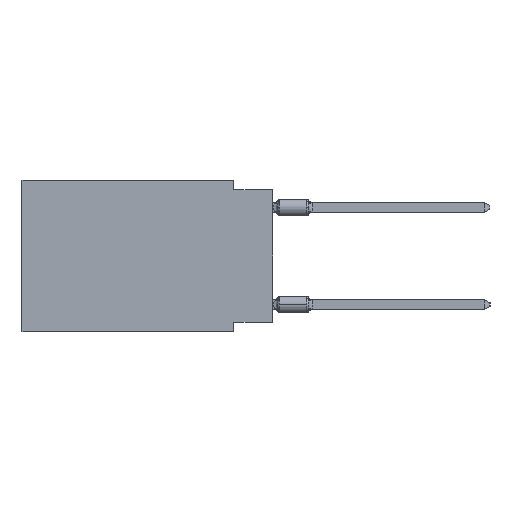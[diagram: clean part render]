
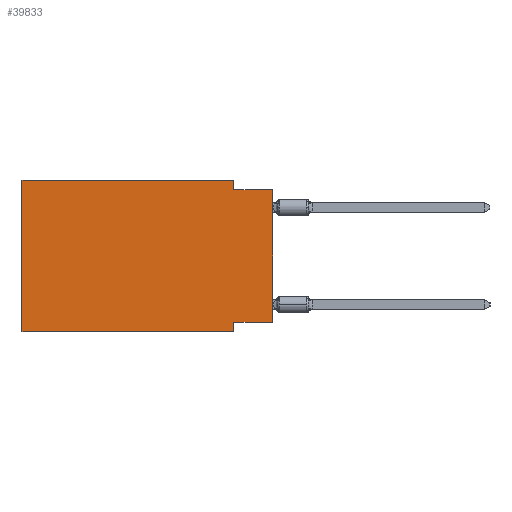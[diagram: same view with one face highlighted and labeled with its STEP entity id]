
A CAD part, left-side view. The second image highlights one B-rep face of the part: STEP entity #39833.
In plain terms, the highlighted planar face has unit normal (-1, 0, 0).
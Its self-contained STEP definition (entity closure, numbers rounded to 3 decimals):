
#191 = DIRECTION ( 'NONE',  ( 0., 0., 1. ) ) ;
#580 = ORIENTED_EDGE ( 'NONE', *, *, #36542, .F. ) ;
#1062 = ORIENTED_EDGE ( 'NONE', *, *, #32069, .F. ) ;
#1510 = FACE_OUTER_BOUND ( 'NONE', #15687, .T. ) ;
#2168 = CARTESIAN_POINT ( 'NONE',  ( 0., 16.383, 0. ) ) ;
#2452 = DIRECTION ( 'NONE',  ( 0., 0., 1. ) ) ;
#4817 = VECTOR ( 'NONE', #40927, 1000. ) ;
#5210 = AXIS2_PLACEMENT_3D ( 'NONE', #20588, #33257, #12476 ) ;
#7306 = DIRECTION ( 'NONE',  ( 0., -1., 0. ) ) ;
#7735 = CARTESIAN_POINT ( 'NONE',  ( 0., 2.54, -9.271 ) ) ;
#8302 = LINE ( 'NONE', #33609, #25710 ) ;
#9130 = VERTEX_POINT ( 'NONE', #20212 ) ;
#11033 = CARTESIAN_POINT ( 'NONE',  ( 0., 16.383, 0. ) ) ;
#11598 = EDGE_CURVE ( 'NONE', #34764, #33278, #39577, .T. ) ;
#11799 = CARTESIAN_POINT ( 'NONE',  ( 0., 0., 0. ) ) ;
#12476 = DIRECTION ( 'NONE',  ( 0., 0., -1. ) ) ;
#12644 = LINE ( 'NONE', #25909, #13486 ) ;
#13308 = ORIENTED_EDGE ( 'NONE', *, *, #27473, .T. ) ;
#13486 = VECTOR ( 'NONE', #191, 1000. ) ;
#14678 = CARTESIAN_POINT ( 'NONE',  ( 0., 2.54, 0. ) ) ;
#14810 = CARTESIAN_POINT ( 'NONE',  ( 0., 16.383, -9.906 ) ) ;
#15114 = LINE ( 'NONE', #11799, #21422 ) ;
#15620 = CARTESIAN_POINT ( 'NONE',  ( 0., 0., -9.271 ) ) ;
#15687 = EDGE_LOOP ( 'NONE', ( #13308, #1062, #30824, #21571, #31313, #17595, #580, #33397 ) ) ;
#16104 = EDGE_CURVE ( 'NONE', #22402, #34764, #26996, .T. ) ;
#16504 = CARTESIAN_POINT ( 'NONE',  ( 0., 0., -9.271 ) ) ;
#16979 = CARTESIAN_POINT ( 'NONE',  ( 0., 2.54, 0. ) ) ;
#17037 = VECTOR ( 'NONE', #30903, 1000. ) ;
#17595 = ORIENTED_EDGE ( 'NONE', *, *, #33598, .T. ) ;
#17702 = CARTESIAN_POINT ( 'NONE',  ( 0., 0., -0.635 ) ) ;
#18030 = VECTOR ( 'NONE', #21095, 1000. ) ;
#20212 = CARTESIAN_POINT ( 'NONE',  ( 0., 2.54, -9.906 ) ) ;
#20588 = CARTESIAN_POINT ( 'NONE',  ( 0., 16.383, 0. ) ) ;
#21095 = DIRECTION ( 'NONE',  ( 0., 0., -1. ) ) ;
#21422 = VECTOR ( 'NONE', #2452, 1000. ) ;
#21571 = ORIENTED_EDGE ( 'NONE', *, *, #16104, .F. ) ;
#21600 = VECTOR ( 'NONE', #7306, 1000. ) ;
#22402 = VERTEX_POINT ( 'NONE', #2168 ) ;
#25710 = VECTOR ( 'NONE', #33818, 1000. ) ;
#25831 = EDGE_CURVE ( 'NONE', #26641, #35912, #28277, .T. ) ;
#25909 = CARTESIAN_POINT ( 'NONE',  ( 0., 16.383, 0. ) ) ;
#26641 = VERTEX_POINT ( 'NONE', #16504 ) ;
#26996 = LINE ( 'NONE', #11033, #21600 ) ;
#27473 = EDGE_CURVE ( 'NONE', #26641, #30458, #15114, .T. ) ;
#27774 = VECTOR ( 'NONE', #29831, 1000. ) ;
#28253 = EDGE_CURVE ( 'NONE', #29119, #22402, #12644, .T. ) ;
#28277 = LINE ( 'NONE', #15620, #4817 ) ;
#28385 = LINE ( 'NONE', #14810, #27774 ) ;
#29119 = VERTEX_POINT ( 'NONE', #29334 ) ;
#29334 = CARTESIAN_POINT ( 'NONE',  ( 0., 16.383, -9.906 ) ) ;
#29831 = DIRECTION ( 'NONE',  ( 0., -1., 0. ) ) ;
#30458 = VERTEX_POINT ( 'NONE', #17702 ) ;
#30824 = ORIENTED_EDGE ( 'NONE', *, *, #11598, .F. ) ;
#30903 = DIRECTION ( 'NONE',  ( 0., 0., -1. ) ) ;
#31313 = ORIENTED_EDGE ( 'NONE', *, *, #28253, .F. ) ;
#32069 = EDGE_CURVE ( 'NONE', #33278, #30458, #8302, .T. ) ;
#33257 = DIRECTION ( 'NONE',  ( 1., 0., 0. ) ) ;
#33278 = VERTEX_POINT ( 'NONE', #36317 ) ;
#33397 = ORIENTED_EDGE ( 'NONE', *, *, #25831, .F. ) ;
#33598 = EDGE_CURVE ( 'NONE', #29119, #9130, #28385, .T. ) ;
#33609 = CARTESIAN_POINT ( 'NONE',  ( 0., 0., -0.635 ) ) ;
#33614 = CARTESIAN_POINT ( 'NONE',  ( 0., 2.54, -9.906 ) ) ;
#33818 = DIRECTION ( 'NONE',  ( 0., -1., 0. ) ) ;
#34764 = VERTEX_POINT ( 'NONE', #16979 ) ;
#35912 = VERTEX_POINT ( 'NONE', #7735 ) ;
#36317 = CARTESIAN_POINT ( 'NONE',  ( 0., 2.54, -0.635 ) ) ;
#36542 = EDGE_CURVE ( 'NONE', #35912, #9130, #36920, .T. ) ;
#36920 = LINE ( 'NONE', #33614, #17037 ) ;
#39477 = PLANE ( 'NONE',  #5210 ) ;
#39577 = LINE ( 'NONE', #14678, #18030 ) ;
#39833 = ADVANCED_FACE ( 'NONE', ( #1510 ), #39477, .F. ) ;
#40927 = DIRECTION ( 'NONE',  ( 0., 1., 0. ) ) ;
